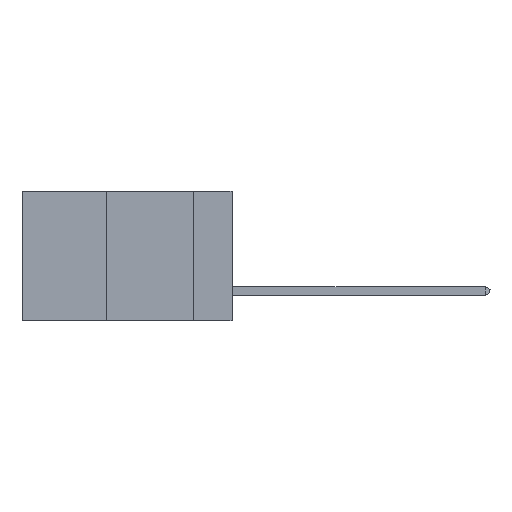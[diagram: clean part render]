
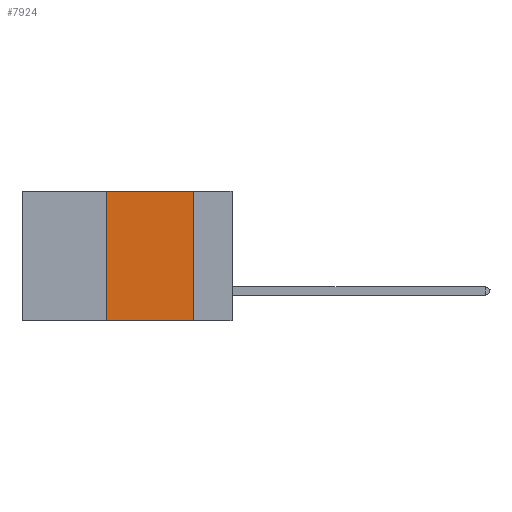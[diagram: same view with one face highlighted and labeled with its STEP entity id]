
A CAD part, left-side view. The second image highlights one B-rep face of the part: STEP entity #7924.
In plain terms, the highlighted planar face has unit normal (-1, 0, 0).
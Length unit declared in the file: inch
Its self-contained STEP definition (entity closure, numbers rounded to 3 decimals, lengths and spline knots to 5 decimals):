
#1205 = VECTOR ( 'NONE', #3089, 39.37008 ) ;
#1914 = CARTESIAN_POINT ( 'NONE',  ( 0., 0.11, 0. ) ) ;
#3089 = DIRECTION ( 'NONE',  ( 0., -1., 0. ) ) ;
#5065 = CARTESIAN_POINT ( 'NONE',  ( 0., 0.36, 0. ) ) ;
#7754 = VERTEX_POINT ( 'NONE', #5065 ) ;
#7924 = ADVANCED_FACE ( 'NONE', ( #15686 ), #23978, .F. ) ;
#8113 = DIRECTION ( 'NONE',  ( 0., 0., -1. ) ) ;
#9348 = ORIENTED_EDGE ( 'NONE', *, *, #29719, .F. ) ;
#9351 = VECTOR ( 'NONE', #10950, 39.37008 ) ;
#9791 = ORIENTED_EDGE ( 'NONE', *, *, #16196, .F. ) ;
#10950 = DIRECTION ( 'NONE',  ( 0., 0., 1. ) ) ;
#12748 = CARTESIAN_POINT ( 'NONE',  ( 0., 0.6, 0. ) ) ;
#14099 = CARTESIAN_POINT ( 'NONE',  ( 0., 0.11, 0. ) ) ;
#15526 = EDGE_CURVE ( 'NONE', #7754, #16857, #16460, .T. ) ;
#15686 = FACE_OUTER_BOUND ( 'NONE', #20811, .T. ) ;
#16196 = EDGE_CURVE ( 'NONE', #36463, #7754, #26974, .T. ) ;
#16460 = LINE ( 'NONE', #33369, #31443 ) ;
#16857 = VERTEX_POINT ( 'NONE', #14099 ) ;
#17767 = ORIENTED_EDGE ( 'NONE', *, *, #15526, .F. ) ;
#19189 = AXIS2_PLACEMENT_3D ( 'NONE', #12748, #36401, #8113 ) ;
#20811 = EDGE_LOOP ( 'NONE', ( #9348, #17767, #9791, #29218 ) ) ;
#21619 = DIRECTION ( 'NONE',  ( 0., 0., -1. ) ) ;
#22172 = LINE ( 'NONE', #1914, #35400 ) ;
#22399 = CARTESIAN_POINT ( 'NONE',  ( 0., 0.36, 0. ) ) ;
#23978 = PLANE ( 'NONE',  #19189 ) ;
#26596 = CARTESIAN_POINT ( 'NONE',  ( 0., 0.36, -0.37 ) ) ;
#26974 = LINE ( 'NONE', #22399, #9351 ) ;
#27596 = DIRECTION ( 'NONE',  ( 0., -1., 0. ) ) ;
#29218 = ORIENTED_EDGE ( 'NONE', *, *, #30464, .T. ) ;
#29719 = EDGE_CURVE ( 'NONE', #16857, #35802, #22172, .T. ) ;
#30464 = EDGE_CURVE ( 'NONE', #36463, #35802, #33337, .T. ) ;
#31443 = VECTOR ( 'NONE', #27596, 39.37008 ) ;
#33337 = LINE ( 'NONE', #34235, #1205 ) ;
#33369 = CARTESIAN_POINT ( 'NONE',  ( 0., 0.6, 0. ) ) ;
#34235 = CARTESIAN_POINT ( 'NONE',  ( 0., 0.6, -0.37 ) ) ;
#35153 = CARTESIAN_POINT ( 'NONE',  ( 0., 0.11, -0.37 ) ) ;
#35400 = VECTOR ( 'NONE', #21619, 39.37008 ) ;
#35802 = VERTEX_POINT ( 'NONE', #35153 ) ;
#36401 = DIRECTION ( 'NONE',  ( 1., 0., 0. ) ) ;
#36463 = VERTEX_POINT ( 'NONE', #26596 ) ;
